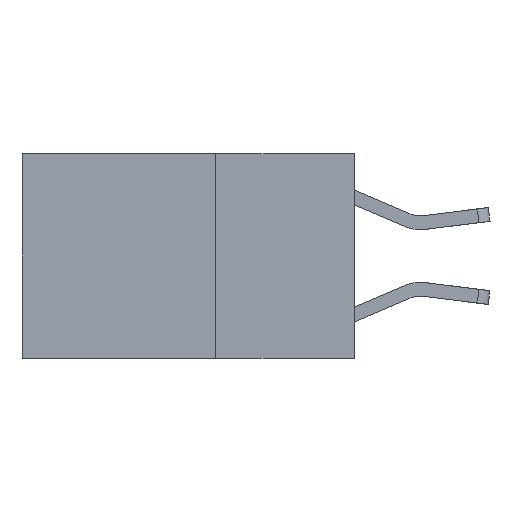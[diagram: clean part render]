
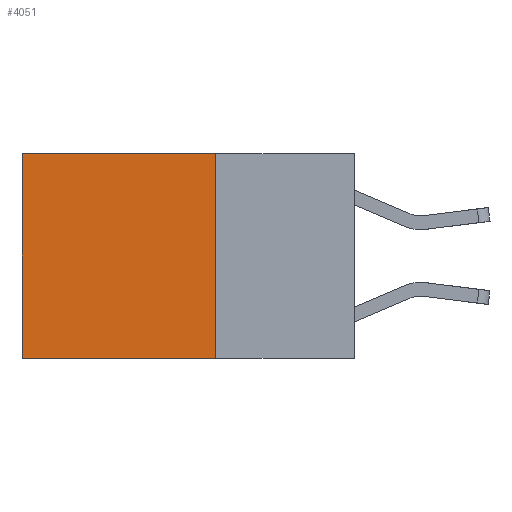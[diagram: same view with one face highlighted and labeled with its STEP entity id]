
A CAD part, left-side view. The second image highlights one B-rep face of the part: STEP entity #4051.
In plain terms, the highlighted planar face has unit normal (-1, 0, 0).
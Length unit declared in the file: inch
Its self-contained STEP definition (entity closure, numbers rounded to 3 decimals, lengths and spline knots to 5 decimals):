
#66 = EDGE_CURVE ( 'NONE', #9093, #2294, #5795, .T. ) ;
#896 = DIRECTION ( 'NONE',  ( 0., 1., 0. ) ) ;
#1364 = DIRECTION ( 'NONE',  ( 1., 0., 0. ) ) ;
#1834 = EDGE_LOOP ( 'NONE', ( #9143, #11011, #1890, #8649 ) ) ;
#1889 = CARTESIAN_POINT ( 'NONE',  ( 0.2625, 0.6, -0.37 ) ) ;
#1890 = ORIENTED_EDGE ( 'NONE', *, *, #66, .F. ) ;
#2294 = VERTEX_POINT ( 'NONE', #11358 ) ;
#2307 = CARTESIAN_POINT ( 'NONE',  ( 0.2625, 0.25, 0. ) ) ;
#2615 = EDGE_CURVE ( 'NONE', #4880, #8978, #6899, .T. ) ;
#2974 = CARTESIAN_POINT ( 'NONE',  ( 0.2625, 0.25, 0. ) ) ;
#3036 = VECTOR ( 'NONE', #9990, 39.37008 ) ;
#3300 = PLANE ( 'NONE',  #8946 ) ;
#3776 = VECTOR ( 'NONE', #896, 39.37008 ) ;
#4051 = ADVANCED_FACE ( 'NONE', ( #8531 ), #3300, .F. ) ;
#4603 = DIRECTION ( 'NONE',  ( 0., 0., -1. ) ) ;
#4805 = CARTESIAN_POINT ( 'NONE',  ( 0.2625, 0.25, 0. ) ) ;
#4880 = VERTEX_POINT ( 'NONE', #10991 ) ;
#4933 = VECTOR ( 'NONE', #4603, 39.37008 ) ;
#5149 = DIRECTION ( 'NONE',  ( 0., 1., 0. ) ) ;
#5552 = EDGE_CURVE ( 'NONE', #2294, #8978, #8006, .T. ) ;
#5795 = LINE ( 'NONE', #7451, #3036 ) ;
#5809 = VECTOR ( 'NONE', #5149, 39.37008 ) ;
#6150 = LINE ( 'NONE', #4805, #3776 ) ;
#6899 = LINE ( 'NONE', #7163, #4933 ) ;
#7163 = CARTESIAN_POINT ( 'NONE',  ( 0.2625, 0.6, 0. ) ) ;
#7451 = CARTESIAN_POINT ( 'NONE',  ( 0.2625, 0.25, 0. ) ) ;
#7705 = DIRECTION ( 'NONE',  ( 0., 0., -1. ) ) ;
#8006 = LINE ( 'NONE', #9235, #5809 ) ;
#8531 = FACE_OUTER_BOUND ( 'NONE', #1834, .T. ) ;
#8649 = ORIENTED_EDGE ( 'NONE', *, *, #11220, .T. ) ;
#8946 = AXIS2_PLACEMENT_3D ( 'NONE', #2307, #1364, #7705 ) ;
#8978 = VERTEX_POINT ( 'NONE', #1889 ) ;
#9093 = VERTEX_POINT ( 'NONE', #2974 ) ;
#9143 = ORIENTED_EDGE ( 'NONE', *, *, #2615, .T. ) ;
#9235 = CARTESIAN_POINT ( 'NONE',  ( 0.2625, 0.25, -0.37 ) ) ;
#9990 = DIRECTION ( 'NONE',  ( 0., 0., -1. ) ) ;
#10991 = CARTESIAN_POINT ( 'NONE',  ( 0.2625, 0.6, 0. ) ) ;
#11011 = ORIENTED_EDGE ( 'NONE', *, *, #5552, .F. ) ;
#11220 = EDGE_CURVE ( 'NONE', #9093, #4880, #6150, .T. ) ;
#11358 = CARTESIAN_POINT ( 'NONE',  ( 0.2625, 0.25, -0.37 ) ) ;
